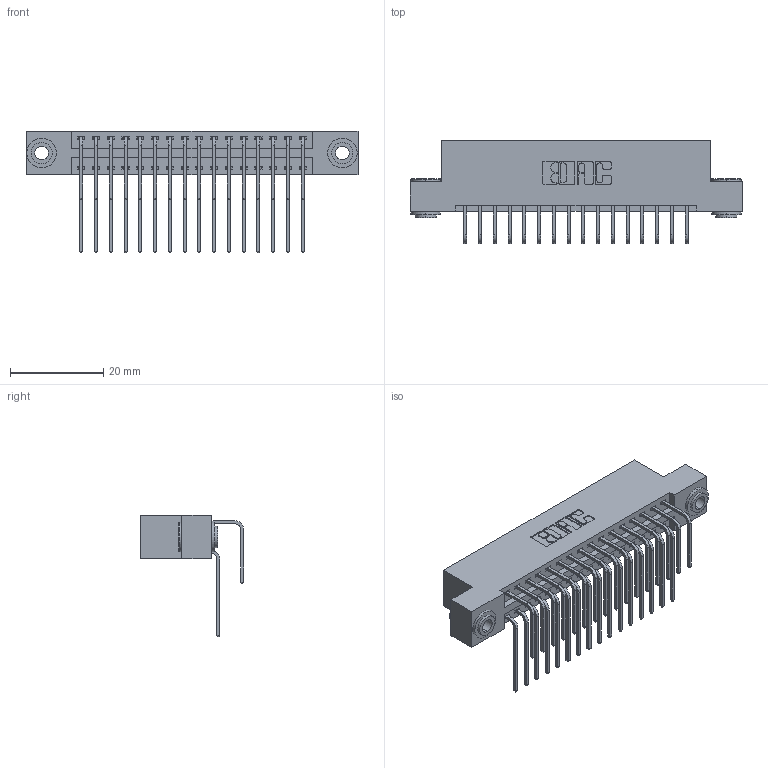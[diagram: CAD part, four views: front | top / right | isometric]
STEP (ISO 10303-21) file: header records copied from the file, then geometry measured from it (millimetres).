
FILE_DESCRIPTION (( 'STEP AP203' ), '1' );
FILE_NAME ('346-032-558-203.STEP', '2022-05-19T18:32:38', ( '' ), ( '' ), 'SwSTEP 2.0', 'SolidWorks 2020', '' );
FILE_SCHEMA (( 'CONFIG_CONTROL_DESIGN' ));
Length unit declared in the file: inch
Products named in the file (5): 346-032-558-203; 346 Part_Flush Mounting Lugs - 0.156 Dia-TH; 345-250-002_345-250-002-102; 345-292-001_558 Tail - 2; 345-292-001_558 559 Tail - 1
Assembly tree (35 placements, depth 2):
  346-032-558-203
    346 Part_Flush Mounting Lugs - 0.156 Dia-TH
    345-292-001_558 559 Tail - 1  x16
    345-292-001_558 Tail - 2  x16
    345-250-002_345-250-002-102  x2
Bounding box: 71.37 x 22.16 x 26.16 mm (x, y, z)
Volume: 6943.8 mm3; surface area: 10270.4 mm2
Topology: 35 solids, 35 shells, 1902 faces, 5593 edges, 3682 vertices
Faces by surface type: plane 1284, cylinder 610, cone 8
Entity records: 16792 total; most frequent: CARTESIAN_POINT 2836, ORIENTED_EDGE 2710, DIRECTION 2553, EDGE_CURVE 1355, VECTOR 1095, LINE 1095, VERTEX_POINT 898, AXIS2_PLACEMENT_3D 729
